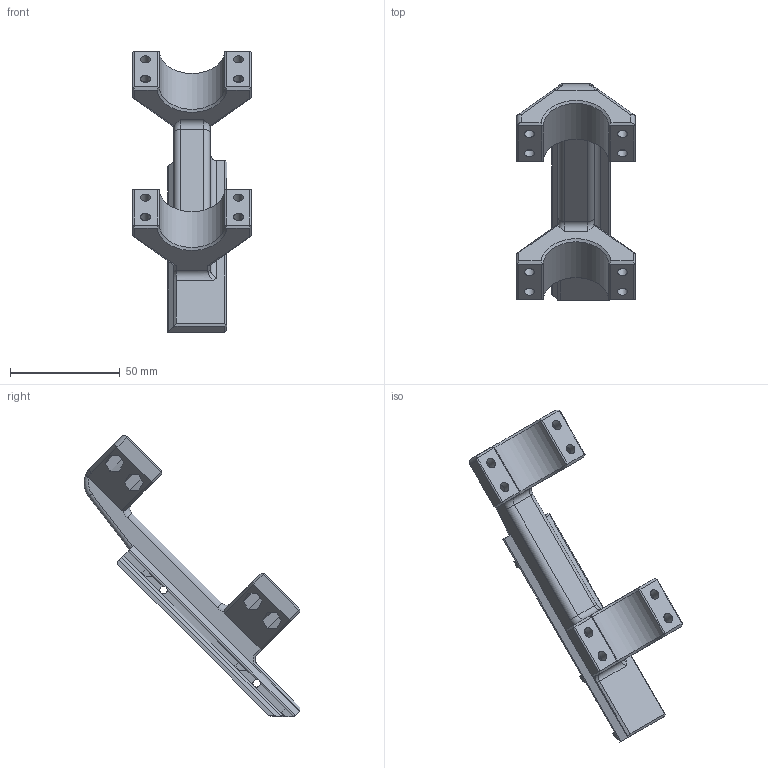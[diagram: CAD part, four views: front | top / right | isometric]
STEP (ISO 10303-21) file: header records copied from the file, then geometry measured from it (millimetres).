
FILE_DESCRIPTION(/* description */ (''),/* implementation_level */ '2;1');
FILE_NAME(/* name */ 'LPL Body - 1.47in.step',/* time_stamp */ '2022-10-12T08:52:15-05:00',/* author */ (''),/* organization */ (''),/* preprocessor_version */ 'ST-DEVELOPER v19',/* originating_system */ 'Autodesk Translation Framework v11.7.0.108',/* authorisation */ '');
FILE_SCHEMA (('AUTOMOTIVE_DESIGN { 1 0 10303 214 3 1 1 }'));
Length unit declared in the file: millimetre
Products named in the file (1): LPL Optic Mount
Bounding box: 54 x 98.37 x 128.19 mm (x, y, z)
Volume: 64222.6 mm3; surface area: 21753.2 mm2
Topology: 1 solids, 1 shells, 211 faces, 575 edges, 374 vertices
Faces by surface type: plane 158, cylinder 35, bspline 7, torus 6, cone 5
Full cylindrical faces by diameter (mm): 4.5 x8
Entity records: 7171 total; most frequent: CARTESIAN_POINT 1802, ORIENTED_EDGE 1150, DIRECTION 1030, EDGE_CURVE 575, LINE 442, VECTOR 442, VERTEX_POINT 374, AXIS2_PLACEMENT_3D 294
